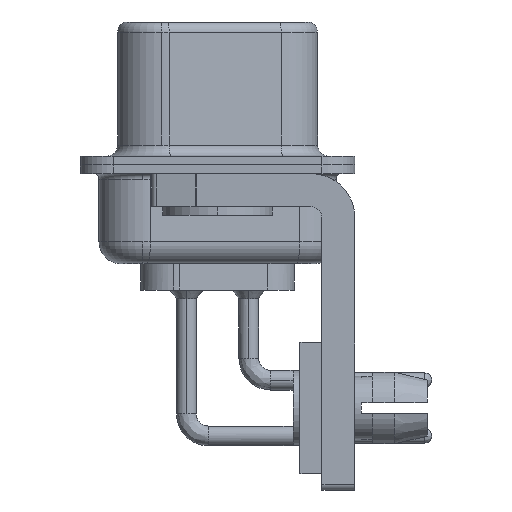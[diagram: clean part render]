
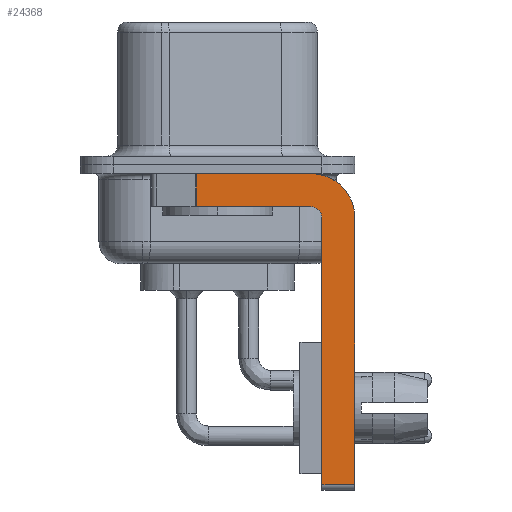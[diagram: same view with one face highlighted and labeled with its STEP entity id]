
A CAD part, left-side view. The second image highlights one B-rep face of the part: STEP entity #24368.
In plain terms, the highlighted planar face has unit normal (-1, 0, 0).
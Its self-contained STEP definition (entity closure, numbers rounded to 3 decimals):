
#205 = EDGE_CURVE ( 'NONE', #1833, #11420, #7768, .T. ) ;
#539 = CARTESIAN_POINT ( 'NONE',  ( -2.9, -6.25, -14.55 ) ) ;
#1171 = DIRECTION ( 'NONE',  ( 0., 0., -1. ) ) ;
#1264 = CARTESIAN_POINT ( 'NONE',  ( -2.9, -4.75, -14.55 ) ) ;
#1281 = ORIENTED_EDGE ( 'NONE', *, *, #7797, .F. ) ;
#1282 = LINE ( 'NONE', #9257, #22028 ) ;
#1313 = ORIENTED_EDGE ( 'NONE', *, *, #205, .T. ) ;
#1420 = CARTESIAN_POINT ( 'NONE',  ( -2.9, -4.75, -14.8 ) ) ;
#1541 = VERTEX_POINT ( 'NONE', #3778 ) ;
#1833 = VERTEX_POINT ( 'NONE', #1264 ) ;
#2416 = VECTOR ( 'NONE', #15094, 1000. ) ;
#2812 = ORIENTED_EDGE ( 'NONE', *, *, #14450, .F. ) ;
#2926 = LINE ( 'NONE', #17059, #3562 ) ;
#3015 = DIRECTION ( 'NONE',  ( 0., 1., 0. ) ) ;
#3083 = CIRCLE ( 'NONE', #13310, 2. ) ;
#3361 = DIRECTION ( 'NONE',  ( 0., 0., 1. ) ) ;
#3562 = VECTOR ( 'NONE', #3015, 1000. ) ;
#3623 = ORIENTED_EDGE ( 'NONE', *, *, #13910, .F. ) ;
#3778 = CARTESIAN_POINT ( 'NONE',  ( -2.9, -4.25, -1.9 ) ) ;
#4098 = PLANE ( 'NONE',  #5725 ) ;
#4826 = AXIS2_PLACEMENT_3D ( 'NONE', #6302, #20345, #8310 ) ;
#5573 = VERTEX_POINT ( 'NONE', #9233 ) ;
#5650 = EDGE_CURVE ( 'NONE', #18722, #12694, #3083, .T. ) ;
#5725 = AXIS2_PLACEMENT_3D ( 'NONE', #14050, #18120, #6103 ) ;
#5778 = DIRECTION ( 'NONE',  ( 0., 0., -1. ) ) ;
#6012 = VERTEX_POINT ( 'NONE', #17973 ) ;
#6103 = DIRECTION ( 'NONE',  ( 0., 0., -1. ) ) ;
#6302 = CARTESIAN_POINT ( 'NONE',  ( -2.9, -4.25, -2.4 ) ) ;
#7244 = ORIENTED_EDGE ( 'NONE', *, *, #5650, .F. ) ;
#7768 = LINE ( 'NONE', #15141, #2416 ) ;
#7797 = EDGE_CURVE ( 'NONE', #5573, #1541, #22477, .T. ) ;
#8310 = DIRECTION ( 'NONE',  ( 0., 0., 1. ) ) ;
#9233 = CARTESIAN_POINT ( 'NONE',  ( -2.9, -4.75, -2.4 ) ) ;
#9257 = CARTESIAN_POINT ( 'NONE',  ( -2.9, 0.978, -1.9 ) ) ;
#9623 = CARTESIAN_POINT ( 'NONE',  ( -2.9, 0.978, -0.4 ) ) ;
#9894 = LINE ( 'NONE', #1420, #19332 ) ;
#10217 = ORIENTED_EDGE ( 'NONE', *, *, #10433, .F. ) ;
#10433 = EDGE_CURVE ( 'NONE', #12694, #11420, #17924, .T. ) ;
#11299 = CARTESIAN_POINT ( 'NONE',  ( -2.9, 3., -0.4 ) ) ;
#11420 = VERTEX_POINT ( 'NONE', #539 ) ;
#12629 = VECTOR ( 'NONE', #15329, 1000. ) ;
#12694 = VERTEX_POINT ( 'NONE', #21881 ) ;
#13190 = VECTOR ( 'NONE', #5778, 1000. ) ;
#13310 = AXIS2_PLACEMENT_3D ( 'NONE', #21697, #21525, #21500 ) ;
#13910 = EDGE_CURVE ( 'NONE', #1541, #6012, #2926, .T. ) ;
#13924 = ORIENTED_EDGE ( 'NONE', *, *, #24748, .T. ) ;
#14050 = CARTESIAN_POINT ( 'NONE',  ( -2.9, -4.25, -2.4 ) ) ;
#14450 = EDGE_CURVE ( 'NONE', #24220, #18722, #18008, .T. ) ;
#15094 = DIRECTION ( 'NONE',  ( 0., -1., 0. ) ) ;
#15141 = CARTESIAN_POINT ( 'NONE',  ( -2.9, -4.25, -14.55 ) ) ;
#15329 = DIRECTION ( 'NONE',  ( 0., -1., 0. ) ) ;
#16847 = ORIENTED_EDGE ( 'NONE', *, *, #21624, .F. ) ;
#17059 = CARTESIAN_POINT ( 'NONE',  ( -2.9, -4.25, -1.9 ) ) ;
#17924 = LINE ( 'NONE', #19829, #13190 ) ;
#17973 = CARTESIAN_POINT ( 'NONE',  ( -2.9, 0.978, -1.9 ) ) ;
#18008 = LINE ( 'NONE', #11299, #12629 ) ;
#18120 = DIRECTION ( 'NONE',  ( 1., 0., 0. ) ) ;
#18722 = VERTEX_POINT ( 'NONE', #19154 ) ;
#19154 = CARTESIAN_POINT ( 'NONE',  ( -2.9, -4.25, -0.4 ) ) ;
#19332 = VECTOR ( 'NONE', #3361, 1000. ) ;
#19521 = FACE_OUTER_BOUND ( 'NONE', #24197, .T. ) ;
#19829 = CARTESIAN_POINT ( 'NONE',  ( -2.9, -6.25, -2.4 ) ) ;
#20345 = DIRECTION ( 'NONE',  ( -1., 0., 0. ) ) ;
#21500 = DIRECTION ( 'NONE',  ( 0., 0., -1. ) ) ;
#21525 = DIRECTION ( 'NONE',  ( 1., 0., 0. ) ) ;
#21624 = EDGE_CURVE ( 'NONE', #1833, #5573, #9894, .T. ) ;
#21697 = CARTESIAN_POINT ( 'NONE',  ( -2.9, -4.25, -2.4 ) ) ;
#21881 = CARTESIAN_POINT ( 'NONE',  ( -2.9, -6.25, -2.4 ) ) ;
#22028 = VECTOR ( 'NONE', #1171, 1000. ) ;
#22477 = CIRCLE ( 'NONE', #4826, 0.5 ) ;
#24197 = EDGE_LOOP ( 'NONE', ( #2812, #13924, #3623, #1281, #16847, #1313, #10217, #7244 ) ) ;
#24220 = VERTEX_POINT ( 'NONE', #9623 ) ;
#24368 = ADVANCED_FACE ( 'NONE', ( #19521 ), #4098, .F. ) ;
#24748 = EDGE_CURVE ( 'NONE', #24220, #6012, #1282, .T. ) ;
